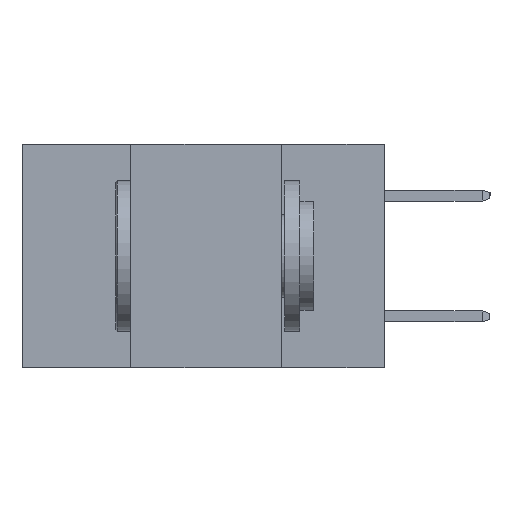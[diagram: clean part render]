
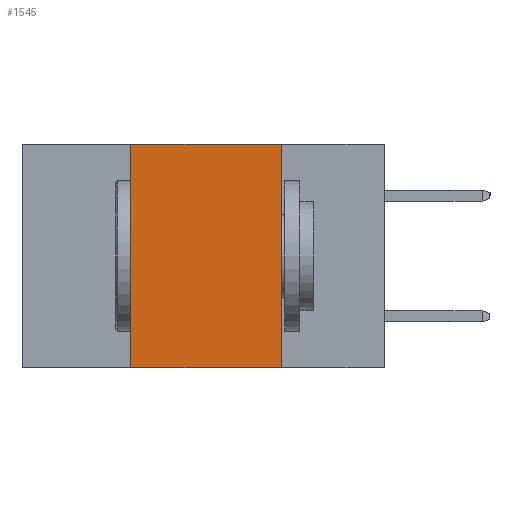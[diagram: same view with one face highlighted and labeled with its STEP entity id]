
A CAD part, left-side view. The second image highlights one B-rep face of the part: STEP entity #1545.
In plain terms, the highlighted planar face has unit normal (-1, 0, 0).
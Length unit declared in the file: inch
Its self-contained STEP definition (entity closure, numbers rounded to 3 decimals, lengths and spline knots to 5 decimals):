
#1495 = VECTOR ( 'NONE', #3540, 39.37008 ) ;
#1545 = ADVANCED_FACE ( 'NONE', ( #2701 ), #7307, .F. ) ;
#1868 = CARTESIAN_POINT ( 'NONE',  ( 0., 0.6, 0. ) ) ;
#1955 = EDGE_CURVE ( 'NONE', #12297, #16094, #13380, .T. ) ;
#2065 = CARTESIAN_POINT ( 'NONE',  ( 0., 0.42, -0.37 ) ) ;
#2697 = CARTESIAN_POINT ( 'NONE',  ( 0., 0.17, 0. ) ) ;
#2701 = FACE_OUTER_BOUND ( 'NONE', #4777, .T. ) ;
#3540 = DIRECTION ( 'NONE',  ( 0., -1., 0. ) ) ;
#3752 = LINE ( 'NONE', #1868, #1495 ) ;
#4777 = EDGE_LOOP ( 'NONE', ( #16944, #19893, #14880, #11335 ) ) ;
#4966 = EDGE_CURVE ( 'NONE', #20242, #13198, #17108, .T. ) ;
#5107 = DIRECTION ( 'NONE',  ( 0., 0., 1. ) ) ;
#5849 = DIRECTION ( 'NONE',  ( 1., 0., 0. ) ) ;
#5944 = CARTESIAN_POINT ( 'NONE',  ( 0., 0.17, -0.37 ) ) ;
#7232 = VECTOR ( 'NONE', #13967, 39.37008 ) ;
#7307 = PLANE ( 'NONE',  #20485 ) ;
#8461 = EDGE_CURVE ( 'NONE', #16094, #20242, #3752, .T. ) ;
#8887 = DIRECTION ( 'NONE',  ( 0., 0., -1. ) ) ;
#8997 = LINE ( 'NONE', #12154, #20367 ) ;
#9056 = CARTESIAN_POINT ( 'NONE',  ( 0., 0.42, -0.37 ) ) ;
#10800 = VECTOR ( 'NONE', #5107, 39.37008 ) ;
#11335 = ORIENTED_EDGE ( 'NONE', *, *, #17200, .T. ) ;
#12154 = CARTESIAN_POINT ( 'NONE',  ( 0., 0.6, -0.37 ) ) ;
#12297 = VERTEX_POINT ( 'NONE', #9056 ) ;
#13198 = VERTEX_POINT ( 'NONE', #5944 ) ;
#13380 = LINE ( 'NONE', #2065, #10800 ) ;
#13967 = DIRECTION ( 'NONE',  ( 0., 0., -1. ) ) ;
#14037 = DIRECTION ( 'NONE',  ( 0., -1., 0. ) ) ;
#14754 = CARTESIAN_POINT ( 'NONE',  ( 0., 0.42, 0. ) ) ;
#14880 = ORIENTED_EDGE ( 'NONE', *, *, #1955, .F. ) ;
#15384 = CARTESIAN_POINT ( 'NONE',  ( 0., 0.6, 0. ) ) ;
#16094 = VERTEX_POINT ( 'NONE', #14754 ) ;
#16794 = CARTESIAN_POINT ( 'NONE',  ( 0., 0.17, -0.37 ) ) ;
#16944 = ORIENTED_EDGE ( 'NONE', *, *, #4966, .F. ) ;
#17108 = LINE ( 'NONE', #16794, #7232 ) ;
#17200 = EDGE_CURVE ( 'NONE', #12297, #13198, #8997, .T. ) ;
#19893 = ORIENTED_EDGE ( 'NONE', *, *, #8461, .F. ) ;
#20242 = VERTEX_POINT ( 'NONE', #2697 ) ;
#20367 = VECTOR ( 'NONE', #14037, 39.37008 ) ;
#20485 = AXIS2_PLACEMENT_3D ( 'NONE', #15384, #5849, #8887 ) ;
